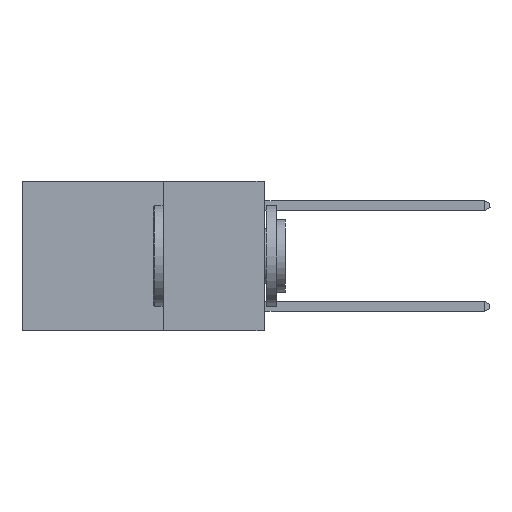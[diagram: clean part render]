
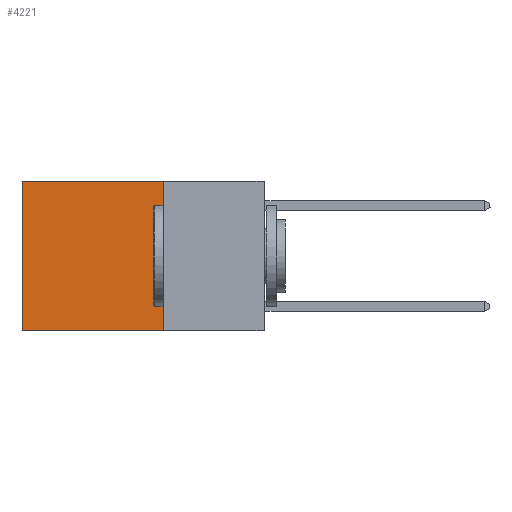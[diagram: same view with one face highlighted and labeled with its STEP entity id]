
A CAD part, left-side view. The second image highlights one B-rep face of the part: STEP entity #4221.
In plain terms, the highlighted planar face has unit normal (-1, 0, 0).
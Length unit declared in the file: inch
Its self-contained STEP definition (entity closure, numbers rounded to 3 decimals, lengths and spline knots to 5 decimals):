
#1065 = VECTOR ( 'NONE', #14921, 39.37008 ) ;
#1556 = CARTESIAN_POINT ( 'NONE',  ( 0.2625, 0.25, 0. ) ) ;
#2127 = DIRECTION ( 'NONE',  ( 1., 0., 0. ) ) ;
#2219 = LINE ( 'NONE', #1556, #17522 ) ;
#2592 = EDGE_CURVE ( 'NONE', #6360, #4797, #9863, .T. ) ;
#3104 = LINE ( 'NONE', #3277, #11494 ) ;
#3277 = CARTESIAN_POINT ( 'NONE',  ( 0.2625, 0.25, -0.37 ) ) ;
#3562 = CARTESIAN_POINT ( 'NONE',  ( 0.2625, 0.25, 0. ) ) ;
#4221 = ADVANCED_FACE ( 'NONE', ( #13390 ), #18427, .F. ) ;
#4421 = AXIS2_PLACEMENT_3D ( 'NONE', #3562, #2127, #12464 ) ;
#4587 = CARTESIAN_POINT ( 'NONE',  ( 0.2625, 0.6, 0. ) ) ;
#4797 = VERTEX_POINT ( 'NONE', #4853 ) ;
#4853 = CARTESIAN_POINT ( 'NONE',  ( 0.2625, 0.6, 0. ) ) ;
#6360 = VERTEX_POINT ( 'NONE', #14262 ) ;
#7734 = ORIENTED_EDGE ( 'NONE', *, *, #19076, .F. ) ;
#8337 = VERTEX_POINT ( 'NONE', #8934 ) ;
#8934 = CARTESIAN_POINT ( 'NONE',  ( 0.2625, 0.25, -0.37 ) ) ;
#9091 = EDGE_CURVE ( 'NONE', #4797, #17416, #12439, .T. ) ;
#9863 = LINE ( 'NONE', #11979, #17671 ) ;
#10324 = ORIENTED_EDGE ( 'NONE', *, *, #2592, .T. ) ;
#11017 = EDGE_CURVE ( 'NONE', #8337, #17416, #3104, .T. ) ;
#11494 = VECTOR ( 'NONE', #13609, 39.37008 ) ;
#11913 = DIRECTION ( 'NONE',  ( 0., 1., 0. ) ) ;
#11979 = CARTESIAN_POINT ( 'NONE',  ( 0.2625, 0.25, 0. ) ) ;
#12439 = LINE ( 'NONE', #4587, #1065 ) ;
#12464 = DIRECTION ( 'NONE',  ( 0., 0., -1. ) ) ;
#13390 = FACE_OUTER_BOUND ( 'NONE', #14626, .T. ) ;
#13402 = DIRECTION ( 'NONE',  ( 0., 0., -1. ) ) ;
#13609 = DIRECTION ( 'NONE',  ( 0., 1., 0. ) ) ;
#13901 = ORIENTED_EDGE ( 'NONE', *, *, #9091, .T. ) ;
#14221 = CARTESIAN_POINT ( 'NONE',  ( 0.2625, 0.6, -0.37 ) ) ;
#14262 = CARTESIAN_POINT ( 'NONE',  ( 0.2625, 0.25, 0. ) ) ;
#14626 = EDGE_LOOP ( 'NONE', ( #13901, #15701, #7734, #10324 ) ) ;
#14921 = DIRECTION ( 'NONE',  ( 0., 0., -1. ) ) ;
#15701 = ORIENTED_EDGE ( 'NONE', *, *, #11017, .F. ) ;
#17416 = VERTEX_POINT ( 'NONE', #14221 ) ;
#17522 = VECTOR ( 'NONE', #13402, 39.37008 ) ;
#17671 = VECTOR ( 'NONE', #11913, 39.37008 ) ;
#18427 = PLANE ( 'NONE',  #4421 ) ;
#19076 = EDGE_CURVE ( 'NONE', #6360, #8337, #2219, .T. ) ;
